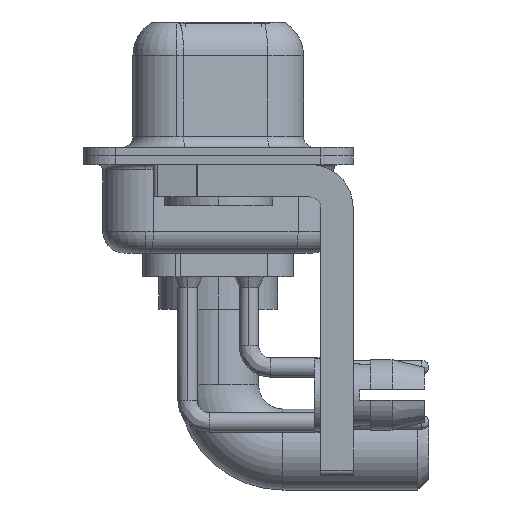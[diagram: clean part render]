
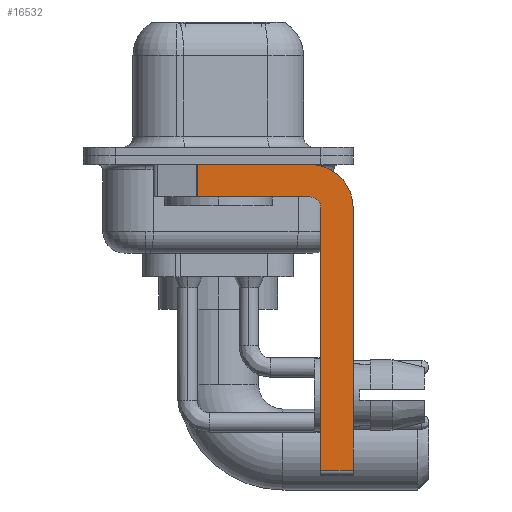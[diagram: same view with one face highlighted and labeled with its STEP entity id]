
A CAD part, left-side view. The second image highlights one B-rep face of the part: STEP entity #16532.
In plain terms, the highlighted planar face has unit normal (-1, 0, 0).
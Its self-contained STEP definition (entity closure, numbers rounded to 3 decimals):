
#112 = VERTEX_POINT ( 'NONE', #2918 ) ;
#945 = PLANE ( 'NONE',  #3522 ) ;
#2039 = EDGE_CURVE ( 'NONE', #17187, #112, #8766, .T. ) ;
#2171 = LINE ( 'NONE', #11791, #5681 ) ;
#2632 = CARTESIAN_POINT ( 'NONE',  ( -2.9, -6.25, -14.55 ) ) ;
#2918 = CARTESIAN_POINT ( 'NONE',  ( -2.9, -4.25, -0.4 ) ) ;
#3522 = AXIS2_PLACEMENT_3D ( 'NONE', #24255, #16263, #6995 ) ;
#3655 = VECTOR ( 'NONE', #20449, 1000. ) ;
#3734 = VERTEX_POINT ( 'NONE', #20610 ) ;
#4142 = ORIENTED_EDGE ( 'NONE', *, *, #9011, .T. ) ;
#4271 = DIRECTION ( 'NONE',  ( 0., 1., 0. ) ) ;
#4805 = VERTEX_POINT ( 'NONE', #23033 ) ;
#4989 = EDGE_CURVE ( 'NONE', #14771, #3734, #15921, .T. ) ;
#5439 = AXIS2_PLACEMENT_3D ( 'NONE', #18922, #12839, #24768 ) ;
#5523 = VECTOR ( 'NONE', #10162, 1000. ) ;
#5660 = EDGE_CURVE ( 'NONE', #112, #4805, #19625, .T. ) ;
#5681 = VECTOR ( 'NONE', #11550, 1000. ) ;
#5824 = EDGE_CURVE ( 'NONE', #23151, #14771, #9897, .T. ) ;
#6487 = CARTESIAN_POINT ( 'NONE',  ( -2.9, 0.978, -1.9 ) ) ;
#6995 = DIRECTION ( 'NONE',  ( 0., 0., -1. ) ) ;
#7585 = VECTOR ( 'NONE', #14935, 1000. ) ;
#8273 = ORIENTED_EDGE ( 'NONE', *, *, #20516, .F. ) ;
#8766 = LINE ( 'NONE', #10673, #3655 ) ;
#8872 = VERTEX_POINT ( 'NONE', #16259 ) ;
#9011 = EDGE_CURVE ( 'NONE', #17187, #3734, #19811, .T. ) ;
#9897 = CIRCLE ( 'NONE', #20027, 0.5 ) ;
#10162 = DIRECTION ( 'NONE',  ( 0., 0., -1. ) ) ;
#10673 = CARTESIAN_POINT ( 'NONE',  ( -2.9, 3., -0.4 ) ) ;
#10958 = DIRECTION ( 'NONE',  ( 0., 0., 1. ) ) ;
#11348 = ORIENTED_EDGE ( 'NONE', *, *, #2039, .F. ) ;
#11550 = DIRECTION ( 'NONE',  ( 0., -1., 0. ) ) ;
#11791 = CARTESIAN_POINT ( 'NONE',  ( -2.9, -4.25, -14.55 ) ) ;
#12321 = CARTESIAN_POINT ( 'NONE',  ( -2.9, -4.75, -2.4 ) ) ;
#12839 = DIRECTION ( 'NONE',  ( 1., 0., 0. ) ) ;
#13283 = EDGE_CURVE ( 'NONE', #8872, #23532, #2171, .T. ) ;
#14771 = VERTEX_POINT ( 'NONE', #19687 ) ;
#14935 = DIRECTION ( 'NONE',  ( 0., 0., -1. ) ) ;
#15251 = EDGE_LOOP ( 'NONE', ( #11348, #4142, #20083, #15855, #8273, #21211, #23267, #22407 ) ) ;
#15855 = ORIENTED_EDGE ( 'NONE', *, *, #5824, .F. ) ;
#15857 = DIRECTION ( 'NONE',  ( 0., 0., 1. ) ) ;
#15921 = LINE ( 'NONE', #19989, #21595 ) ;
#16259 = CARTESIAN_POINT ( 'NONE',  ( -2.9, -4.75, -14.55 ) ) ;
#16263 = DIRECTION ( 'NONE',  ( 1., 0., 0. ) ) ;
#16532 = ADVANCED_FACE ( 'NONE', ( #18787 ), #945, .F. ) ;
#17176 = EDGE_CURVE ( 'NONE', #4805, #23532, #22812, .T. ) ;
#17187 = VERTEX_POINT ( 'NONE', #22681 ) ;
#17647 = DIRECTION ( 'NONE',  ( -1., 0., 0. ) ) ;
#18787 = FACE_OUTER_BOUND ( 'NONE', #15251, .T. ) ;
#18922 = CARTESIAN_POINT ( 'NONE',  ( -2.9, -4.25, -2.4 ) ) ;
#19409 = VECTOR ( 'NONE', #10958, 1000. ) ;
#19625 = CIRCLE ( 'NONE', #5439, 2. ) ;
#19687 = CARTESIAN_POINT ( 'NONE',  ( -2.9, -4.25, -1.9 ) ) ;
#19811 = LINE ( 'NONE', #6487, #5523 ) ;
#19989 = CARTESIAN_POINT ( 'NONE',  ( -2.9, -4.25, -1.9 ) ) ;
#20027 = AXIS2_PLACEMENT_3D ( 'NONE', #21208, #17647, #15857 ) ;
#20083 = ORIENTED_EDGE ( 'NONE', *, *, #4989, .F. ) ;
#20449 = DIRECTION ( 'NONE',  ( 0., -1., 0. ) ) ;
#20516 = EDGE_CURVE ( 'NONE', #8872, #23151, #22502, .T. ) ;
#20595 = CARTESIAN_POINT ( 'NONE',  ( -2.9, -4.75, -14.8 ) ) ;
#20610 = CARTESIAN_POINT ( 'NONE',  ( -2.9, 0.978, -1.9 ) ) ;
#21034 = CARTESIAN_POINT ( 'NONE',  ( -2.9, -6.25, -2.4 ) ) ;
#21208 = CARTESIAN_POINT ( 'NONE',  ( -2.9, -4.25, -2.4 ) ) ;
#21211 = ORIENTED_EDGE ( 'NONE', *, *, #13283, .T. ) ;
#21595 = VECTOR ( 'NONE', #4271, 1000. ) ;
#22407 = ORIENTED_EDGE ( 'NONE', *, *, #5660, .F. ) ;
#22502 = LINE ( 'NONE', #20595, #19409 ) ;
#22681 = CARTESIAN_POINT ( 'NONE',  ( -2.9, 0.978, -0.4 ) ) ;
#22812 = LINE ( 'NONE', #21034, #7585 ) ;
#23033 = CARTESIAN_POINT ( 'NONE',  ( -2.9, -6.25, -2.4 ) ) ;
#23151 = VERTEX_POINT ( 'NONE', #12321 ) ;
#23267 = ORIENTED_EDGE ( 'NONE', *, *, #17176, .F. ) ;
#23532 = VERTEX_POINT ( 'NONE', #2632 ) ;
#24255 = CARTESIAN_POINT ( 'NONE',  ( -2.9, -4.25, -2.4 ) ) ;
#24768 = DIRECTION ( 'NONE',  ( 0., 0., -1. ) ) ;
